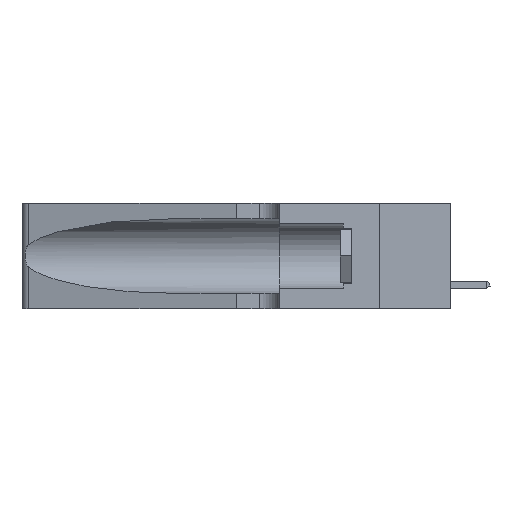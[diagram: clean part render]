
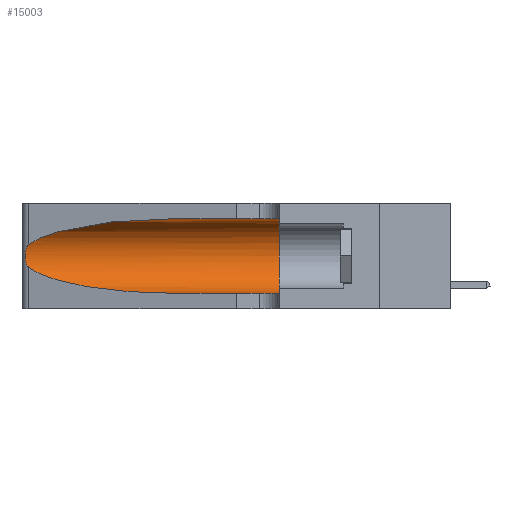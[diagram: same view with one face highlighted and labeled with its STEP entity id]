
A CAD part, left-side view. The second image highlights one B-rep face of the part: STEP entity #15003.
In plain terms, the highlighted cylindrical face has radius 3.308 mm (diameter 6.617 mm), a partial arc.
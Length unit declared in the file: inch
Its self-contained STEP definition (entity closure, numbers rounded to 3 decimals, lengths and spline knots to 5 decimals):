
#75 = EDGE_CURVE ( 'NONE', #35326, #28996, #11777, .T. ) ;
#900 = CARTESIAN_POINT ( 'NONE',  ( 0.1305, 1.61858, 0.05475 ) ) ;
#928 = CARTESIAN_POINT ( 'NONE',  ( 0.1305, 0.72297, 0.05475 ) ) ;
#2077 = ORIENTED_EDGE ( 'NONE', *, *, #11306, .T. ) ;
#2791 = CARTESIAN_POINT ( 'NONE',  ( 0.25789, 1.23486, 0.15765 ) ) ;
#2987 = ORIENTED_EDGE ( 'NONE', *, *, #34697, .T. ) ;
#4250 = CARTESIAN_POINT ( 'NONE',  ( 0.1305, 0.72297, 0.31525 ) ) ;
#5452 = CARTESIAN_POINT ( 'NONE',  ( 0.25856, 1.23593, 0.16098 ) ) ;
#5680 = CARTESIAN_POINT ( 'NONE',  ( 0.25555, 1.22993, 0.14849 ) ) ;
#5808 = CARTESIAN_POINT ( 'NONE',  ( 0.25854, 1.2359, 0.20912 ) ) ;
#6706 = CARTESIAN_POINT ( 'NONE',  ( 0.1305, 0.72297, 0.31525 ) ) ;
#8066 = ORIENTED_EDGE ( 'NONE', *, *, #75, .T. ) ;
#8152 = DIRECTION ( 'NONE',  ( 0., -1., 0. ) ) ;
#8612 = CARTESIAN_POINT ( 'NONE',  ( 0.25487, 1.22718, 0.14631 ) ) ;
#9120 = EDGE_CURVE ( 'NONE', #22887, #19846, #12965, .T. ) ;
#10024 = CARTESIAN_POINT ( 'NONE',  ( 0.1305, 0.35, 0.185 ) ) ;
#11306 = EDGE_CURVE ( 'NONE', #28996, #22887, #29163, .T. ) ;
#11499 = EDGE_LOOP ( 'NONE', ( #2987, #8066, #2077, #18022, #21866, #12944 ) ) ;
#11777 = B_SPLINE_CURVE_WITH_KNOTS ( 'NONE', 3,
 ( #22656, #37231, #31296, #19904, #5808, #14182, #37451, #20126, #22998, #5452, #2791, #28872, #5680, #8612 ),
 .UNSPECIFIED., .F., .F.,
 ( 4, 2, 2, 2, 2, 2, 4 ),
 ( 0., 0.00027, 0.00053, 0.00107, 0.0016, 0.00187, 0.00214 ),
 .UNSPECIFIED. ) ;
#12442 =( BOUNDED_CURVE ( )  B_SPLINE_CURVE ( 3, ( #6706, #26694, #26815, #12661 ),
 .UNSPECIFIED., .F., .F. ) 
 B_SPLINE_CURVE_WITH_KNOTS ( ( 4, 4 ),
 ( 1.5708, 2.84003 ),
 .UNSPECIFIED. ) 
 CURVE ( )  GEOMETRIC_REPRESENTATION_ITEM ( )  RATIONAL_B_SPLINE_CURVE ( ( 1., 0.87, 0.87, 1. ) ) 
 REPRESENTATION_ITEM ( '' )  );
#12661 = CARTESIAN_POINT ( 'NONE',  ( 0.25487, 1.22718, 0.22369 ) ) ;
#12944 = ORIENTED_EDGE ( 'NONE', *, *, #33959, .F. ) ;
#12965 = LINE ( 'NONE', #900, #28408 ) ;
#14182 = CARTESIAN_POINT ( 'NONE',  ( 0.26018, 1.23835, 0.19895 ) ) ;
#14795 = CARTESIAN_POINT ( 'NONE',  ( 0.1305, 0.35, 0.31525 ) ) ;
#14843 = CARTESIAN_POINT ( 'NONE',  ( 0.25487, 1.22718, 0.14631 ) ) ;
#15003 = ADVANCED_FACE ( 'NONE', ( #24260 ), #23322, .F. ) ;
#15735 = VERTEX_POINT ( 'NONE', #4250 ) ;
#15871 = DIRECTION ( 'NONE',  ( 0., -1., 0. ) ) ;
#16002 = CARTESIAN_POINT ( 'NONE',  ( 0.1305, 1.61858, 0.185 ) ) ;
#16142 = CARTESIAN_POINT ( 'NONE',  ( 0.25487, 1.22718, 0.14631 ) ) ;
#18022 = ORIENTED_EDGE ( 'NONE', *, *, #9120, .T. ) ;
#18627 = DIRECTION ( 'NONE',  ( 0., 1., 0. ) ) ;
#19846 = VERTEX_POINT ( 'NONE', #31092 ) ;
#19904 = CARTESIAN_POINT ( 'NONE',  ( 0.25787, 1.23484, 0.2124 ) ) ;
#20126 = CARTESIAN_POINT ( 'NONE',  ( 0.26075, 1.23896, 0.178 ) ) ;
#21866 = ORIENTED_EDGE ( 'NONE', *, *, #31385, .F. ) ;
#22656 = CARTESIAN_POINT ( 'NONE',  ( 0.25487, 1.22718, 0.22369 ) ) ;
#22760 = AXIS2_PLACEMENT_3D ( 'NONE', #10024, #18627, #33303 ) ;
#22887 = VERTEX_POINT ( 'NONE', #27720 ) ;
#22998 = CARTESIAN_POINT ( 'NONE',  ( 0.26017, 1.23833, 0.17102 ) ) ;
#23322 = CYLINDRICAL_SURFACE ( 'NONE', #27192, 0.13025 ) ;
#24260 = FACE_OUTER_BOUND ( 'NONE', #11499, .T. ) ;
#24465 = DIRECTION ( 'NONE',  ( 0., 0., -1. ) ) ;
#25583 = VECTOR ( 'NONE', #26606, 39.37008 ) ;
#26606 = DIRECTION ( 'NONE',  ( 0., -1., 0. ) ) ;
#26694 = CARTESIAN_POINT ( 'NONE',  ( 0.18966, 0.96281, 0.31525 ) ) ;
#26815 = CARTESIAN_POINT ( 'NONE',  ( 0.2373, 1.15595, 0.28018 ) ) ;
#27192 = AXIS2_PLACEMENT_3D ( 'NONE', #16002, #15871, #24465 ) ;
#27205 = CARTESIAN_POINT ( 'NONE',  ( 0.25487, 1.22718, 0.22369 ) ) ;
#27402 = LINE ( 'NONE', #34548, #25583 ) ;
#27720 = CARTESIAN_POINT ( 'NONE',  ( 0.1305, 0.72297, 0.05475 ) ) ;
#28408 = VECTOR ( 'NONE', #8152, 39.37008 ) ;
#28872 = CARTESIAN_POINT ( 'NONE',  ( 0.25639, 1.23186, 0.15144 ) ) ;
#28996 = VERTEX_POINT ( 'NONE', #16142 ) ;
#29163 =( BOUNDED_CURVE ( )  B_SPLINE_CURVE ( 3, ( #14843, #32192, #35225, #928 ),
 .UNSPECIFIED., .F., .F. ) 
 B_SPLINE_CURVE_WITH_KNOTS ( ( 4, 4 ),
 ( 3.44316, 4.71239 ),
 .UNSPECIFIED. ) 
 CURVE ( )  GEOMETRIC_REPRESENTATION_ITEM ( )  RATIONAL_B_SPLINE_CURVE ( ( 1., 0.87, 0.87, 1. ) ) 
 REPRESENTATION_ITEM ( '' )  );
#31092 = CARTESIAN_POINT ( 'NONE',  ( 0.1305, 0.35, 0.05475 ) ) ;
#31296 = CARTESIAN_POINT ( 'NONE',  ( 0.25639, 1.23184, 0.21858 ) ) ;
#31385 = EDGE_CURVE ( 'NONE', #35681, #19846, #34476, .T. ) ;
#32192 = CARTESIAN_POINT ( 'NONE',  ( 0.2373, 1.15595, 0.08982 ) ) ;
#33303 = DIRECTION ( 'NONE',  ( 0., 0., 1. ) ) ;
#33959 = EDGE_CURVE ( 'NONE', #15735, #35681, #27402, .T. ) ;
#34476 = CIRCLE ( 'NONE', #22760, 0.13025 ) ;
#34548 = CARTESIAN_POINT ( 'NONE',  ( 0.1305, 1.61858, 0.31525 ) ) ;
#34697 = EDGE_CURVE ( 'NONE', #15735, #35326, #12442, .T. ) ;
#35225 = CARTESIAN_POINT ( 'NONE',  ( 0.18966, 0.96281, 0.05475 ) ) ;
#35326 = VERTEX_POINT ( 'NONE', #27205 ) ;
#35681 = VERTEX_POINT ( 'NONE', #14795 ) ;
#37231 = CARTESIAN_POINT ( 'NONE',  ( 0.25555, 1.22994, 0.2215 ) ) ;
#37451 = CARTESIAN_POINT ( 'NONE',  ( 0.26075, 1.23896, 0.19203 ) ) ;
